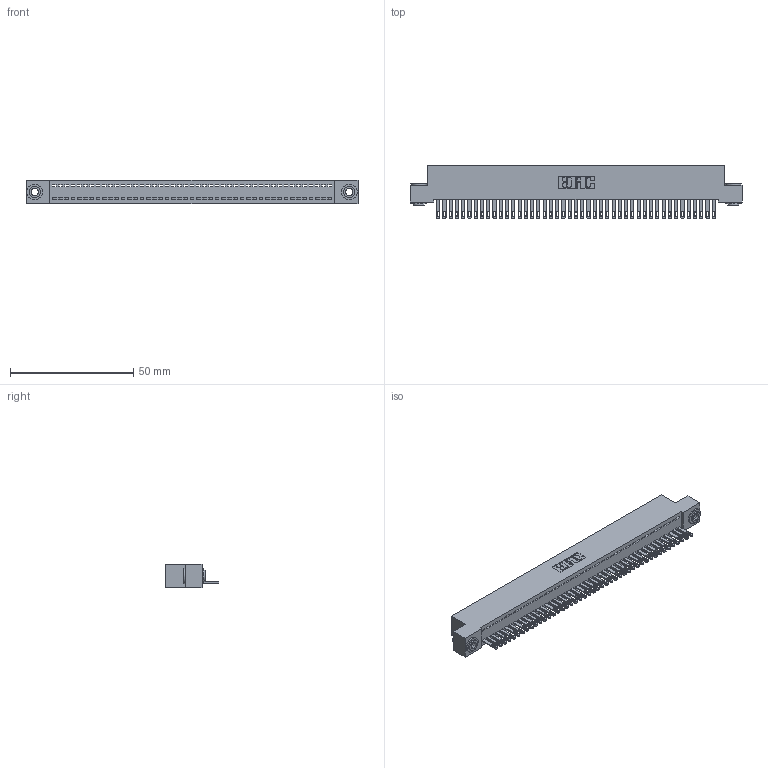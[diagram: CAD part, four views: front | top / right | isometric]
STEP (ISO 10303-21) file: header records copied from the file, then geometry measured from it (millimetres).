
FILE_DESCRIPTION (( 'STEP AP203' ), '1' );
FILE_NAME ('892-045-500-103.STEP', '2020-09-21T17:06:23', ( '' ), ( '' ), 'SwSTEP 2.0', 'SolidWorks 2020', '' );
FILE_SCHEMA (( 'CONFIG_CONTROL_DESIGN' ));
Length unit declared in the file: inch
Products named in the file (4): 842 Part_.156 TH; 345-292-001_345-293-100; 342-250-002_345-250-002-102; 892-045-500-103
Assembly tree (48 placements, depth 2):
  892-045-500-103
    842 Part_.156 TH
    345-292-001_345-293-100  x45
    342-250-002_345-250-002-102  x2
Bounding box: 134.62 x 21.85 x 9.4 mm (x, y, z)
Volume: 11865.2 mm3; surface area: 17794.3 mm2
Topology: 48 solids, 48 shells, 2578 faces, 7935 edges, 5286 vertices
Faces by surface type: plane 1696, cylinder 874, cone 8
Entity records: 27570 total; most frequent: CARTESIAN_POINT 4732, ORIENTED_EDGE 4706, DIRECTION 4021, EDGE_CURVE 2353, VECTOR 2197, LINE 2197, VERTEX_POINT 1566, AXIS2_PLACEMENT_3D 912
